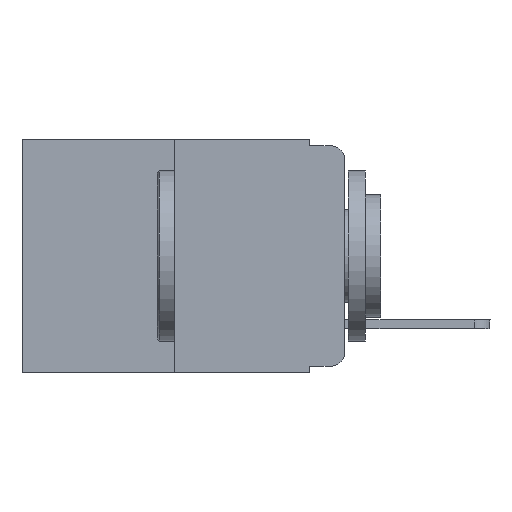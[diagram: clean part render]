
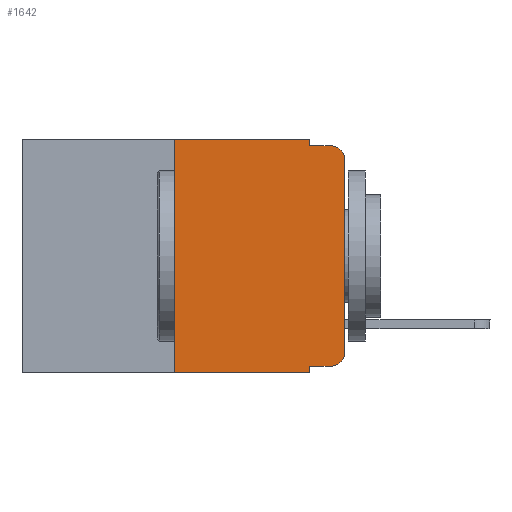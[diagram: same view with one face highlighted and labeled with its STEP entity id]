
A CAD part, left-side view. The second image highlights one B-rep face of the part: STEP entity #1642.
In plain terms, the highlighted planar face has unit normal (-1, 0, 0).
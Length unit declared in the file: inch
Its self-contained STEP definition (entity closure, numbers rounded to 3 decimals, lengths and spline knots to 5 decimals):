
#49 = ORIENTED_EDGE ( 'NONE', *, *, #6603, .T. ) ;
#321 = VERTEX_POINT ( 'NONE', #3387 ) ;
#728 = LINE ( 'NONE', #8845, #5670 ) ;
#1291 = CARTESIAN_POINT ( 'NONE',  ( 0., 0.051, -0.343 ) ) ;
#1356 = VECTOR ( 'NONE', #11488, 39.37008 ) ;
#1551 = LINE ( 'NONE', #4543, #7634 ) ;
#1642 = ADVANCED_FACE ( 'NONE', ( #4663 ), #14376, .F. ) ;
#1714 = AXIS2_PLACEMENT_3D ( 'NONE', #12482, #9403, #13960 ) ;
#2055 = CIRCLE ( 'NONE', #1714, 0.02 ) ;
#2135 = ORIENTED_EDGE ( 'NONE', *, *, #10634, .F. ) ;
#2328 = CARTESIAN_POINT ( 'NONE',  ( 0., 0.473, 0. ) ) ;
#2369 = DIRECTION ( 'NONE',  ( 0., -1., 0. ) ) ;
#2575 = DIRECTION ( 'NONE',  ( 0., 0., -1. ) ) ;
#2638 = LINE ( 'NONE', #7645, #18097 ) ;
#2669 = EDGE_CURVE ( 'NONE', #8806, #4831, #4180, .T. ) ;
#2852 = CARTESIAN_POINT ( 'NONE',  ( 0., 0.02, -0.01 ) ) ;
#2874 = EDGE_LOOP ( 'NONE', ( #49, #16330, #2924, #11877, #2135, #7647, #19260, #2995, #3549, #14002 ) ) ;
#2924 = ORIENTED_EDGE ( 'NONE', *, *, #13782, .F. ) ;
#2995 = ORIENTED_EDGE ( 'NONE', *, *, #9202, .F. ) ;
#3387 = CARTESIAN_POINT ( 'NONE',  ( 0., 0.25, -0.343 ) ) ;
#3549 = ORIENTED_EDGE ( 'NONE', *, *, #18857, .T. ) ;
#3552 = CARTESIAN_POINT ( 'NONE',  ( 0., 0.051, -0.333 ) ) ;
#4180 = LINE ( 'NONE', #12867, #6037 ) ;
#4543 = CARTESIAN_POINT ( 'NONE',  ( 0., 0.25, 0. ) ) ;
#4663 = FACE_OUTER_BOUND ( 'NONE', #2874, .T. ) ;
#4831 = VERTEX_POINT ( 'NONE', #18238 ) ;
#5115 = DIRECTION ( 'NONE',  ( -1., 0., 0. ) ) ;
#5670 = VECTOR ( 'NONE', #11797, 39.37008 ) ;
#5781 = VERTEX_POINT ( 'NONE', #13309 ) ;
#6037 = VECTOR ( 'NONE', #2575, 39.37008 ) ;
#6433 = CARTESIAN_POINT ( 'NONE',  ( 0., 0.051, 0. ) ) ;
#6447 = VERTEX_POINT ( 'NONE', #1291 ) ;
#6603 = EDGE_CURVE ( 'NONE', #18701, #11637, #15190, .T. ) ;
#6737 = VERTEX_POINT ( 'NONE', #16095 ) ;
#6887 = EDGE_CURVE ( 'NONE', #11637, #8064, #2055, .T. ) ;
#7542 = DIRECTION ( 'NONE',  ( 0., 0., 1. ) ) ;
#7634 = VECTOR ( 'NONE', #7542, 39.37008 ) ;
#7645 = CARTESIAN_POINT ( 'NONE',  ( 0., 0.473, -0.343 ) ) ;
#7647 = ORIENTED_EDGE ( 'NONE', *, *, #13214, .F. ) ;
#8011 = CARTESIAN_POINT ( 'NONE',  ( 0., 0.473, 0. ) ) ;
#8064 = VERTEX_POINT ( 'NONE', #2852 ) ;
#8321 = EDGE_CURVE ( 'NONE', #5781, #18701, #18672, .T. ) ;
#8332 = LINE ( 'NONE', #17490, #18885 ) ;
#8485 = CARTESIAN_POINT ( 'NONE',  ( 0., 0.051, 0. ) ) ;
#8672 = DIRECTION ( 'NONE',  ( 0., -1., 0. ) ) ;
#8806 = VERTEX_POINT ( 'NONE', #8485 ) ;
#8845 = CARTESIAN_POINT ( 'NONE',  ( 0., 0.051, -0.333 ) ) ;
#9034 = AXIS2_PLACEMENT_3D ( 'NONE', #17219, #5115, #9730 ) ;
#9202 = EDGE_CURVE ( 'NONE', #15070, #6447, #17391, .T. ) ;
#9310 = DIRECTION ( 'NONE',  ( 0., -1., 0. ) ) ;
#9403 = DIRECTION ( 'NONE',  ( -1., 0., 0. ) ) ;
#9730 = DIRECTION ( 'NONE',  ( 0., 0., -1. ) ) ;
#9996 = CARTESIAN_POINT ( 'NONE',  ( 0., 0., 0. ) ) ;
#10634 = EDGE_CURVE ( 'NONE', #6737, #8806, #10830, .T. ) ;
#10830 = LINE ( 'NONE', #8011, #11512 ) ;
#11488 = DIRECTION ( 'NONE',  ( 0., 0., 1. ) ) ;
#11512 = VECTOR ( 'NONE', #8672, 39.37008 ) ;
#11637 = VERTEX_POINT ( 'NONE', #16875 ) ;
#11797 = DIRECTION ( 'NONE',  ( 0., -1., 0. ) ) ;
#11877 = ORIENTED_EDGE ( 'NONE', *, *, #2669, .F. ) ;
#12482 = CARTESIAN_POINT ( 'NONE',  ( 0., 0.02, -0.03 ) ) ;
#12867 = CARTESIAN_POINT ( 'NONE',  ( 0., 0.051, 0. ) ) ;
#13214 = EDGE_CURVE ( 'NONE', #321, #6737, #1551, .T. ) ;
#13309 = CARTESIAN_POINT ( 'NONE',  ( 0., 0.02, -0.333 ) ) ;
#13782 = EDGE_CURVE ( 'NONE', #4831, #8064, #8332, .T. ) ;
#13960 = DIRECTION ( 'NONE',  ( 0., 0., -1. ) ) ;
#14002 = ORIENTED_EDGE ( 'NONE', *, *, #8321, .T. ) ;
#14376 = PLANE ( 'NONE',  #17521 ) ;
#15070 = VERTEX_POINT ( 'NONE', #3552 ) ;
#15190 = LINE ( 'NONE', #9996, #1356 ) ;
#15808 = DIRECTION ( 'NONE',  ( 0., 0., -1. ) ) ;
#16095 = CARTESIAN_POINT ( 'NONE',  ( 0., 0.25, 0. ) ) ;
#16330 = ORIENTED_EDGE ( 'NONE', *, *, #6887, .T. ) ;
#16875 = CARTESIAN_POINT ( 'NONE',  ( 0., 0., -0.03 ) ) ;
#17219 = CARTESIAN_POINT ( 'NONE',  ( 0., 0.02, -0.313 ) ) ;
#17271 = CARTESIAN_POINT ( 'NONE',  ( 0., 0., -0.313 ) ) ;
#17391 = LINE ( 'NONE', #6433, #17655 ) ;
#17490 = CARTESIAN_POINT ( 'NONE',  ( 0., 0.051, -0.01 ) ) ;
#17519 = DIRECTION ( 'NONE',  ( 1., 0., 0. ) ) ;
#17521 = AXIS2_PLACEMENT_3D ( 'NONE', #2328, #17519, #15808 ) ;
#17655 = VECTOR ( 'NONE', #18615, 39.37008 ) ;
#18097 = VECTOR ( 'NONE', #9310, 39.37008 ) ;
#18238 = CARTESIAN_POINT ( 'NONE',  ( 0., 0.051, -0.01 ) ) ;
#18403 = EDGE_CURVE ( 'NONE', #321, #6447, #2638, .T. ) ;
#18615 = DIRECTION ( 'NONE',  ( 0., 0., -1. ) ) ;
#18672 = CIRCLE ( 'NONE', #9034, 0.02 ) ;
#18701 = VERTEX_POINT ( 'NONE', #17271 ) ;
#18857 = EDGE_CURVE ( 'NONE', #15070, #5781, #728, .T. ) ;
#18885 = VECTOR ( 'NONE', #2369, 39.37008 ) ;
#19260 = ORIENTED_EDGE ( 'NONE', *, *, #18403, .T. ) ;
